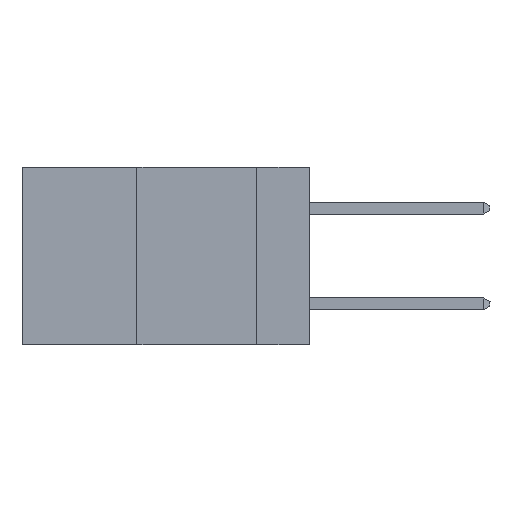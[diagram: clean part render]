
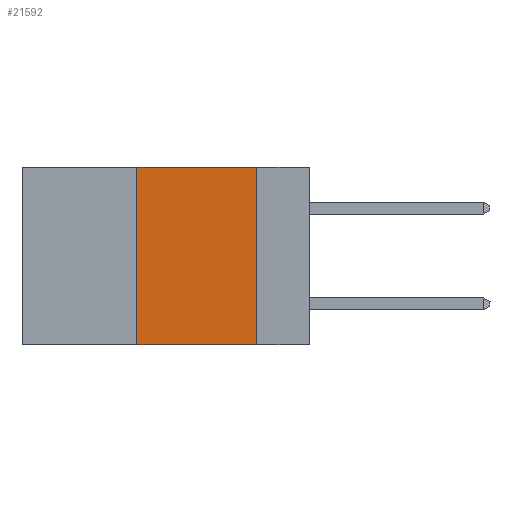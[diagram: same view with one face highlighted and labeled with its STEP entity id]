
A CAD part, left-side view. The second image highlights one B-rep face of the part: STEP entity #21592.
In plain terms, the highlighted planar face has unit normal (-1, 0, 0).
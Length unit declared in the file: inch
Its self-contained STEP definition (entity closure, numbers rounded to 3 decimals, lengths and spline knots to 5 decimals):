
#9 = VECTOR ( 'NONE', #35315, 39.37008 ) ;
#491 = CARTESIAN_POINT ( 'NONE',  ( 0., 0.11, -0.37 ) ) ;
#2471 = DIRECTION ( 'NONE',  ( 1., 0., 0. ) ) ;
#4904 = PLANE ( 'NONE',  #29593 ) ;
#6032 = CARTESIAN_POINT ( 'NONE',  ( 0., 0.6, 0. ) ) ;
#6186 = EDGE_CURVE ( 'NONE', #27903, #12378, #34153, .T. ) ;
#8032 = CARTESIAN_POINT ( 'NONE',  ( 0., 0.11, 0. ) ) ;
#8689 = CARTESIAN_POINT ( 'NONE',  ( 0., 0.6, -0.37 ) ) ;
#9033 = DIRECTION ( 'NONE',  ( 0., 0., -1. ) ) ;
#9156 = FACE_OUTER_BOUND ( 'NONE', #21802, .T. ) ;
#9244 = LINE ( 'NONE', #15514, #33166 ) ;
#10390 = VERTEX_POINT ( 'NONE', #8032 ) ;
#11288 = VECTOR ( 'NONE', #12456, 39.37008 ) ;
#11426 = ORIENTED_EDGE ( 'NONE', *, *, #20475, .F. ) ;
#12378 = VERTEX_POINT ( 'NONE', #491 ) ;
#12456 = DIRECTION ( 'NONE',  ( 0., 0., -1. ) ) ;
#12457 = ORIENTED_EDGE ( 'NONE', *, *, #33126, .F. ) ;
#15514 = CARTESIAN_POINT ( 'NONE',  ( 0., 0.36, 0. ) ) ;
#15811 = VERTEX_POINT ( 'NONE', #30759 ) ;
#16421 = LINE ( 'NONE', #35385, #11288 ) ;
#18984 = CARTESIAN_POINT ( 'NONE',  ( 0., 0.6, 0. ) ) ;
#19861 = CARTESIAN_POINT ( 'NONE',  ( 0., 0.36, -0.37 ) ) ;
#20475 = EDGE_CURVE ( 'NONE', #27903, #15811, #9244, .T. ) ;
#21592 = ADVANCED_FACE ( 'NONE', ( #9156 ), #4904, .F. ) ;
#21802 = EDGE_LOOP ( 'NONE', ( #12457, #25541, #11426, #21963 ) ) ;
#21963 = ORIENTED_EDGE ( 'NONE', *, *, #6186, .T. ) ;
#22241 = DIRECTION ( 'NONE',  ( 0., -1., 0. ) ) ;
#22411 = EDGE_CURVE ( 'NONE', #15811, #10390, #40210, .T. ) ;
#23882 = VECTOR ( 'NONE', #22241, 39.37008 ) ;
#25541 = ORIENTED_EDGE ( 'NONE', *, *, #22411, .F. ) ;
#25591 = DIRECTION ( 'NONE',  ( 0., 0., 1. ) ) ;
#27903 = VERTEX_POINT ( 'NONE', #19861 ) ;
#29593 = AXIS2_PLACEMENT_3D ( 'NONE', #6032, #2471, #9033 ) ;
#30759 = CARTESIAN_POINT ( 'NONE',  ( 0., 0.36, 0. ) ) ;
#33126 = EDGE_CURVE ( 'NONE', #10390, #12378, #16421, .T. ) ;
#33166 = VECTOR ( 'NONE', #25591, 39.37008 ) ;
#34153 = LINE ( 'NONE', #8689, #9 ) ;
#35315 = DIRECTION ( 'NONE',  ( 0., -1., 0. ) ) ;
#35385 = CARTESIAN_POINT ( 'NONE',  ( 0., 0.11, 0. ) ) ;
#40210 = LINE ( 'NONE', #18984, #23882 ) ;
